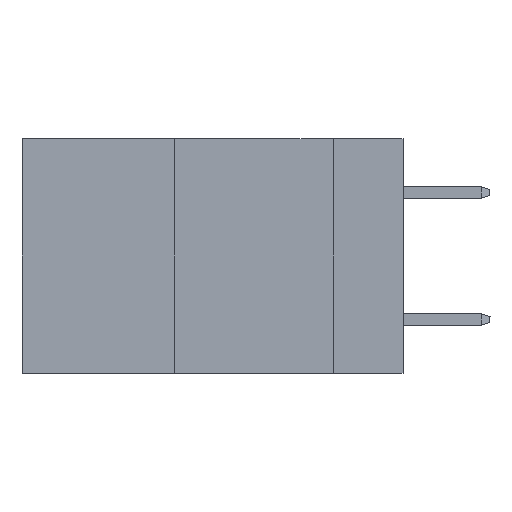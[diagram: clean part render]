
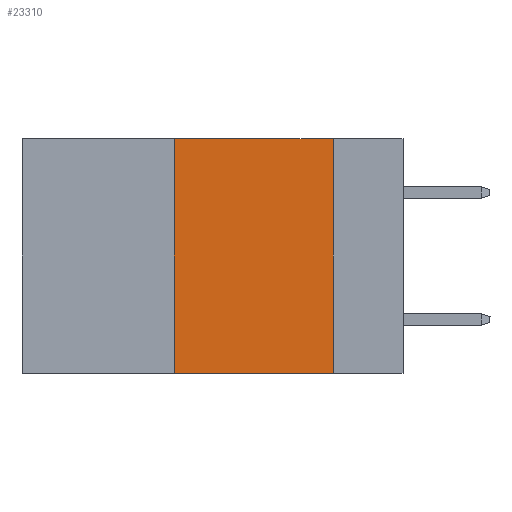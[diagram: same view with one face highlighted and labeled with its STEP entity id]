
A CAD part, left-side view. The second image highlights one B-rep face of the part: STEP entity #23310.
In plain terms, the highlighted planar face has unit normal (-1, 0, 0).
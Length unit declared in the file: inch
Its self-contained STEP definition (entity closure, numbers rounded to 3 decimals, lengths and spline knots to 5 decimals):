
#5 = CARTESIAN_POINT ( 'NONE',  ( 0., 0.36, -0.37 ) ) ;
#189 = VECTOR ( 'NONE', #30792, 39.37008 ) ;
#396 = PLANE ( 'NONE',  #23842 ) ;
#1425 = ORIENTED_EDGE ( 'NONE', *, *, #17654, .F. ) ;
#2023 = LINE ( 'NONE', #17593, #22031 ) ;
#2725 = DIRECTION ( 'NONE',  ( 0., -1., 0. ) ) ;
#2960 = FACE_OUTER_BOUND ( 'NONE', #30797, .T. ) ;
#3134 = CARTESIAN_POINT ( 'NONE',  ( 0., 0.6, 0. ) ) ;
#7000 = DIRECTION ( 'NONE',  ( 0., 0., -1. ) ) ;
#7212 = EDGE_CURVE ( 'NONE', #16135, #25218, #17967, .T. ) ;
#8813 = ORIENTED_EDGE ( 'NONE', *, *, #17025, .F. ) ;
#9476 = CARTESIAN_POINT ( 'NONE',  ( 0., 0.6, 0. ) ) ;
#10837 = DIRECTION ( 'NONE',  ( 1., 0., 0. ) ) ;
#11537 = DIRECTION ( 'NONE',  ( 0., -1., 0. ) ) ;
#11890 = CARTESIAN_POINT ( 'NONE',  ( 0., 0.36, 0. ) ) ;
#13039 = VERTEX_POINT ( 'NONE', #20291 ) ;
#13572 = DIRECTION ( 'NONE',  ( 0., 0., -1. ) ) ;
#14824 = VECTOR ( 'NONE', #11537, 39.37008 ) ;
#15017 = VECTOR ( 'NONE', #2725, 39.37008 ) ;
#15020 = EDGE_CURVE ( 'NONE', #13039, #31222, #17330, .T. ) ;
#16135 = VERTEX_POINT ( 'NONE', #5 ) ;
#17025 = EDGE_CURVE ( 'NONE', #31222, #25218, #2023, .T. ) ;
#17330 = LINE ( 'NONE', #9476, #14824 ) ;
#17593 = CARTESIAN_POINT ( 'NONE',  ( 0., 0.11, 0. ) ) ;
#17654 = EDGE_CURVE ( 'NONE', #16135, #13039, #22453, .T. ) ;
#17967 = LINE ( 'NONE', #23399, #15017 ) ;
#20291 = CARTESIAN_POINT ( 'NONE',  ( 0., 0.36, 0. ) ) ;
#21123 = ORIENTED_EDGE ( 'NONE', *, *, #15020, .F. ) ;
#22031 = VECTOR ( 'NONE', #7000, 39.37008 ) ;
#22195 = CARTESIAN_POINT ( 'NONE',  ( 0., 0.11, 0. ) ) ;
#22453 = LINE ( 'NONE', #11890, #189 ) ;
#23310 = ADVANCED_FACE ( 'NONE', ( #2960 ), #396, .F. ) ;
#23399 = CARTESIAN_POINT ( 'NONE',  ( 0., 0.6, -0.37 ) ) ;
#23842 = AXIS2_PLACEMENT_3D ( 'NONE', #3134, #10837, #13572 ) ;
#25218 = VERTEX_POINT ( 'NONE', #25754 ) ;
#25754 = CARTESIAN_POINT ( 'NONE',  ( 0., 0.11, -0.37 ) ) ;
#30289 = ORIENTED_EDGE ( 'NONE', *, *, #7212, .T. ) ;
#30792 = DIRECTION ( 'NONE',  ( 0., 0., 1. ) ) ;
#30797 = EDGE_LOOP ( 'NONE', ( #8813, #21123, #1425, #30289 ) ) ;
#31222 = VERTEX_POINT ( 'NONE', #22195 ) ;
